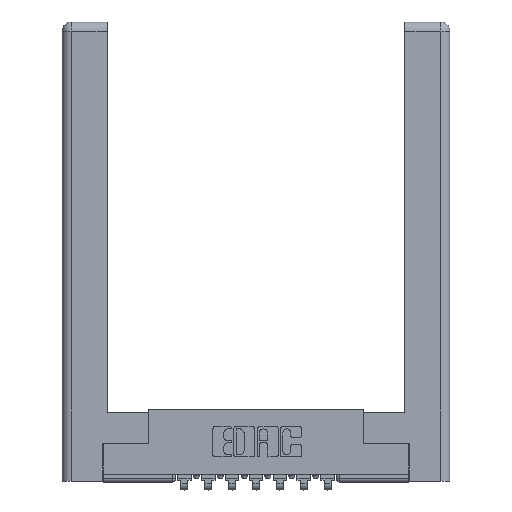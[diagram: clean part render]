
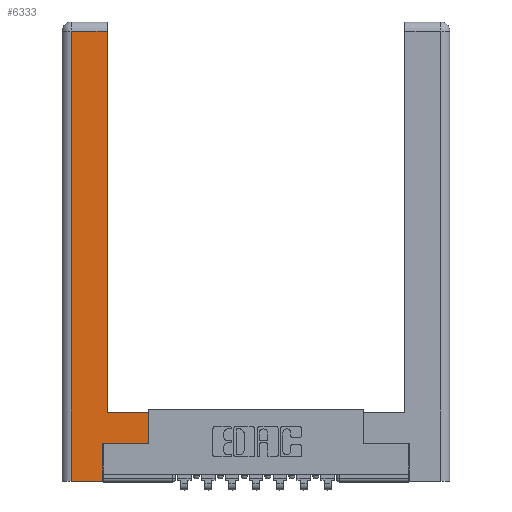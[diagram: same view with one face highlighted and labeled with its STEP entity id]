
A CAD part, top view. The second image highlights one B-rep face of the part: STEP entity #6333.
In plain terms, the highlighted planar face has unit normal (0, 0, 1).
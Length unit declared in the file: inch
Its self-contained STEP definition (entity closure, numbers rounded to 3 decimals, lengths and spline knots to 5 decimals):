
#157 = VECTOR ( 'NONE', #5730, 39.37008 ) ;
#275 = CARTESIAN_POINT ( 'NONE',  ( 0.265, 0.245, 0. ) ) ;
#752 = AXIS2_PLACEMENT_3D ( 'NONE', #1814, #10341, #12440 ) ;
#1117 = ORIENTED_EDGE ( 'NONE', *, *, #10708, .T. ) ;
#1477 = EDGE_CURVE ( 'NONE', #13234, #4276, #12982, .T. ) ;
#1633 = CARTESIAN_POINT ( 'NONE',  ( 0.565, 0.45, 0. ) ) ;
#1814 = CARTESIAN_POINT ( 'NONE',  ( 0., 0., 0. ) ) ;
#2304 = VECTOR ( 'NONE', #3681, 39.37008 ) ;
#2442 = LINE ( 'NONE', #6718, #5363 ) ;
#2969 = DIRECTION ( 'NONE',  ( 0., -1., 0. ) ) ;
#3198 = LINE ( 'NONE', #10892, #10195 ) ;
#3210 = ORIENTED_EDGE ( 'NONE', *, *, #8292, .T. ) ;
#3681 = DIRECTION ( 'NONE',  ( 1., 0., 0. ) ) ;
#3887 = CARTESIAN_POINT ( 'NONE',  ( 0.565, 0.245, 0. ) ) ;
#4226 = CARTESIAN_POINT ( 'NONE',  ( 0.295, 0.45, 0. ) ) ;
#4276 = VERTEX_POINT ( 'NONE', #11564 ) ;
#4644 = ORIENTED_EDGE ( 'NONE', *, *, #6488, .T. ) ;
#4765 = EDGE_CURVE ( 'NONE', #8927, #4996, #3198, .T. ) ;
#4810 = LINE ( 'NONE', #10959, #7977 ) ;
#4826 = DIRECTION ( 'NONE',  ( -1., 0., 0. ) ) ;
#4927 = EDGE_CURVE ( 'NONE', #8885, #10675, #4810, .T. ) ;
#4996 = VERTEX_POINT ( 'NONE', #3887 ) ;
#5063 = ORIENTED_EDGE ( 'NONE', *, *, #9445, .T. ) ;
#5363 = VECTOR ( 'NONE', #4826, 39.37008 ) ;
#5532 = LINE ( 'NONE', #6650, #157 ) ;
#5730 = DIRECTION ( 'NONE',  ( -1., 0., 0. ) ) ;
#5808 = FACE_OUTER_BOUND ( 'NONE', #10466, .T. ) ;
#5964 = VECTOR ( 'NONE', #2969, 39.37008 ) ;
#6127 = LINE ( 'NONE', #8354, #5964 ) ;
#6333 = ADVANCED_FACE ( 'NONE', ( #5808 ), #8179, .F. ) ;
#6397 = ORIENTED_EDGE ( 'NONE', *, *, #4765, .T. ) ;
#6488 = EDGE_CURVE ( 'NONE', #4996, #11091, #7758, .T. ) ;
#6638 = CARTESIAN_POINT ( 'NONE',  ( 0.0615, 0., 0. ) ) ;
#6650 = CARTESIAN_POINT ( 'NONE',  ( 0.0615, 2.94, 0. ) ) ;
#6718 = CARTESIAN_POINT ( 'NONE',  ( 0.295, 0.45, 0. ) ) ;
#7737 = ORIENTED_EDGE ( 'NONE', *, *, #9455, .T. ) ;
#7758 = LINE ( 'NONE', #1633, #11025 ) ;
#7773 = VECTOR ( 'NONE', #12226, 39.37008 ) ;
#7977 = VECTOR ( 'NONE', #9068, 39.37008 ) ;
#8179 = PLANE ( 'NONE',  #752 ) ;
#8292 = EDGE_CURVE ( 'NONE', #13264, #13234, #6127, .T. ) ;
#8354 = CARTESIAN_POINT ( 'NONE',  ( 0.0615, 0., 0. ) ) ;
#8751 = LINE ( 'NONE', #275, #7773 ) ;
#8885 = VERTEX_POINT ( 'NONE', #4226 ) ;
#8927 = VERTEX_POINT ( 'NONE', #13082 ) ;
#8991 = CARTESIAN_POINT ( 'NONE',  ( 0.0615, 2.94, 0. ) ) ;
#9068 = DIRECTION ( 'NONE',  ( 0., 1., 0. ) ) ;
#9183 = ORIENTED_EDGE ( 'NONE', *, *, #4927, .T. ) ;
#9445 = EDGE_CURVE ( 'NONE', #4276, #8927, #8751, .T. ) ;
#9455 = EDGE_CURVE ( 'NONE', #10675, #13264, #5532, .T. ) ;
#9925 = CARTESIAN_POINT ( 'NONE',  ( 0.295, 2.94, 0. ) ) ;
#10195 = VECTOR ( 'NONE', #13824, 39.37008 ) ;
#10341 = DIRECTION ( 'NONE',  ( 0., 0., -1. ) ) ;
#10466 = EDGE_LOOP ( 'NONE', ( #9183, #7737, #3210, #13813, #5063, #6397, #4644, #1117 ) ) ;
#10675 = VERTEX_POINT ( 'NONE', #9925 ) ;
#10708 = EDGE_CURVE ( 'NONE', #11091, #8885, #2442, .T. ) ;
#10760 = DIRECTION ( 'NONE',  ( 0., 1., 0. ) ) ;
#10892 = CARTESIAN_POINT ( 'NONE',  ( 0.565, 0.245, 0. ) ) ;
#10959 = CARTESIAN_POINT ( 'NONE',  ( 0.295, 3., 0. ) ) ;
#11025 = VECTOR ( 'NONE', #10760, 39.37008 ) ;
#11091 = VERTEX_POINT ( 'NONE', #11165 ) ;
#11165 = CARTESIAN_POINT ( 'NONE',  ( 0.565, 0.45, 0. ) ) ;
#11564 = CARTESIAN_POINT ( 'NONE',  ( 0.265, 0., 0. ) ) ;
#12226 = DIRECTION ( 'NONE',  ( 0., 1., 0. ) ) ;
#12440 = DIRECTION ( 'NONE',  ( -1., 0., 0. ) ) ;
#12982 = LINE ( 'NONE', #13261, #2304 ) ;
#13082 = CARTESIAN_POINT ( 'NONE',  ( 0.265, 0.245, 0. ) ) ;
#13234 = VERTEX_POINT ( 'NONE', #6638 ) ;
#13261 = CARTESIAN_POINT ( 'NONE',  ( 0.265, 0., 0. ) ) ;
#13264 = VERTEX_POINT ( 'NONE', #8991 ) ;
#13813 = ORIENTED_EDGE ( 'NONE', *, *, #1477, .T. ) ;
#13824 = DIRECTION ( 'NONE',  ( 1., 0., 0. ) ) ;
